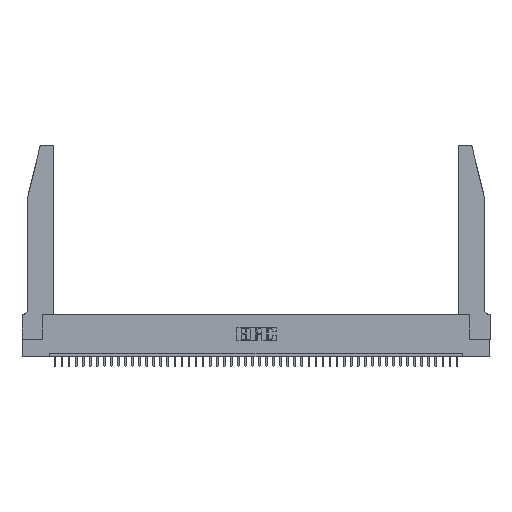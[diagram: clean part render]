
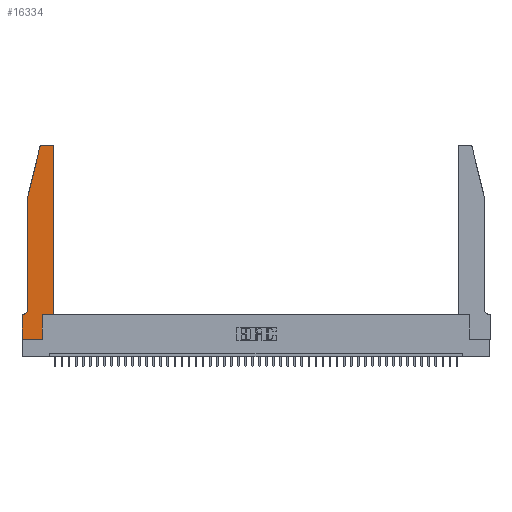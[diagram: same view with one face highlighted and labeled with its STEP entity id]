
A CAD part, top view. The second image highlights one B-rep face of the part: STEP entity #16334.
In plain terms, the highlighted planar face has unit normal (0, 0, 1).
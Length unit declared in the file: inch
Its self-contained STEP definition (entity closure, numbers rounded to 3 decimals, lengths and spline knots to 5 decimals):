
#202 = DIRECTION ( 'NONE',  ( 0., 0., 1. ) ) ;
#338 = CIRCLE ( 'NONE', #2406, 0.03 ) ;
#972 = VECTOR ( 'NONE', #3423, 39.37008 ) ;
#1377 = CARTESIAN_POINT ( 'NONE',  ( 0.2865, 0.35, 0.37 ) ) ;
#1433 = ORIENTED_EDGE ( 'NONE', *, *, #44359, .T. ) ;
#1710 = DIRECTION ( 'NONE',  ( -1., 0., 0. ) ) ;
#1932 = CARTESIAN_POINT ( 'NONE',  ( 0., 0.35, 0.37 ) ) ;
#2041 = CARTESIAN_POINT ( 'NONE',  ( 0.4505, 0.35, 0.37 ) ) ;
#2165 = VECTOR ( 'NONE', #20961, 39.37008 ) ;
#2406 = AXIS2_PLACEMENT_3D ( 'NONE', #21617, #202, #3395 ) ;
#2463 = VERTEX_POINT ( 'NONE', #12196 ) ;
#2534 = CARTESIAN_POINT ( 'NONE',  ( 0., 0., 0.37 ) ) ;
#3395 = DIRECTION ( 'NONE',  ( 1., 0., 0. ) ) ;
#3423 = DIRECTION ( 'NONE',  ( 0., -1., 0. ) ) ;
#3907 = DIRECTION ( 'NONE',  ( -1., 0., 0. ) ) ;
#4202 = DIRECTION ( 'NONE',  ( 1., 0., 0. ) ) ;
#5091 = LINE ( 'NONE', #2041, #32453 ) ;
#5204 = CARTESIAN_POINT ( 'NONE',  ( 0.0755, 2., 0.37 ) ) ;
#5211 = ORIENTED_EDGE ( 'NONE', *, *, #23119, .T. ) ;
#6109 = VERTEX_POINT ( 'NONE', #40522 ) ;
#7480 = LINE ( 'NONE', #2534, #35958 ) ;
#7808 = DIRECTION ( 'NONE',  ( 1., 0., 0. ) ) ;
#8692 = DIRECTION ( 'NONE',  ( 0., 0., 1. ) ) ;
#9276 = DIRECTION ( 'NONE',  ( 0., 1., 0. ) ) ;
#9297 = CARTESIAN_POINT ( 'NONE',  ( 0., 0.35, 0.37 ) ) ;
#9878 = LINE ( 'NONE', #5204, #30496 ) ;
#11547 = EDGE_CURVE ( 'NONE', #17752, #16290, #7480, .T. ) ;
#11912 = DIRECTION ( 'NONE',  ( 0., -1., 0. ) ) ;
#12196 = CARTESIAN_POINT ( 'NONE',  ( 0.4505, 2.72, 0.37 ) ) ;
#12295 = ORIENTED_EDGE ( 'NONE', *, *, #21421, .T. ) ;
#12437 = VERTEX_POINT ( 'NONE', #1377 ) ;
#12793 = CARTESIAN_POINT ( 'NONE',  ( 0.284, 2.72, 0.37 ) ) ;
#13171 = CIRCLE ( 'NONE', #36672, 0.03 ) ;
#13835 = EDGE_CURVE ( 'NONE', #16376, #28984, #25626, .T. ) ;
#14443 = ORIENTED_EDGE ( 'NONE', *, *, #32983, .T. ) ;
#15284 = VERTEX_POINT ( 'NONE', #29966 ) ;
#16290 = VERTEX_POINT ( 'NONE', #25837 ) ;
#16334 = ADVANCED_FACE ( 'NONE', ( #22811 ), #37228, .T. ) ;
#16376 = VERTEX_POINT ( 'NONE', #43990 ) ;
#17752 = VERTEX_POINT ( 'NONE', #31110 ) ;
#18960 = VECTOR ( 'NONE', #21909, 39.37008 ) ;
#19175 = ORIENTED_EDGE ( 'NONE', *, *, #13835, .T. ) ;
#19849 = DIRECTION ( 'NONE',  ( -0.239, -0.971, 0. ) ) ;
#20037 = LINE ( 'NONE', #24501, #972 ) ;
#20463 = CARTESIAN_POINT ( 'NONE',  ( 0.4505, 0.35, 0.37 ) ) ;
#20860 = ORIENTED_EDGE ( 'NONE', *, *, #30473, .T. ) ;
#20961 = DIRECTION ( 'NONE',  ( -1., 0., 0. ) ) ;
#21421 = EDGE_CURVE ( 'NONE', #28984, #17752, #31409, .T. ) ;
#21617 = CARTESIAN_POINT ( 'NONE',  ( 0.4205, 2.72, 0.37 ) ) ;
#21909 = DIRECTION ( 'NONE',  ( 0., 1., 0. ) ) ;
#22383 = EDGE_CURVE ( 'NONE', #44766, #2463, #45265, .T. ) ;
#22584 = EDGE_LOOP ( 'NONE', ( #20860, #5211, #32523, #14443, #23298, #19175, #12295, #41637, #33372, #25308, #46089, #1433 ) ) ;
#22811 = FACE_OUTER_BOUND ( 'NONE', #22584, .T. ) ;
#23119 = EDGE_CURVE ( 'NONE', #30711, #6109, #13171, .T. ) ;
#23289 = DIRECTION ( 'NONE',  ( 1., 0., 0. ) ) ;
#23298 = ORIENTED_EDGE ( 'NONE', *, *, #37552, .T. ) ;
#24154 = VECTOR ( 'NONE', #11912, 39.37008 ) ;
#24501 = CARTESIAN_POINT ( 'NONE',  ( 0.0755, 2., 0.37 ) ) ;
#24625 = LINE ( 'NONE', #43150, #18960 ) ;
#25156 = VECTOR ( 'NONE', #9276, 39.37008 ) ;
#25308 = ORIENTED_EDGE ( 'NONE', *, *, #42397, .T. ) ;
#25626 = LINE ( 'NONE', #35508, #2165 ) ;
#25776 = CARTESIAN_POINT ( 'NONE',  ( 0., 0., 0.37 ) ) ;
#25837 = CARTESIAN_POINT ( 'NONE',  ( 0.2865, 0., 0.37 ) ) ;
#26424 = VERTEX_POINT ( 'NONE', #38576 ) ;
#26479 = EDGE_CURVE ( 'NONE', #16290, #12437, #24625, .T. ) ;
#28166 = LINE ( 'NONE', #28340, #31508 ) ;
#28340 = CARTESIAN_POINT ( 'NONE',  ( 0.2605, 2.75, 0.37 ) ) ;
#28984 = VERTEX_POINT ( 'NONE', #9297 ) ;
#29966 = CARTESIAN_POINT ( 'NONE',  ( 0.4205, 2.75, 0.37 ) ) ;
#30473 = EDGE_CURVE ( 'NONE', #15284, #30711, #28166, .T. ) ;
#30496 = VECTOR ( 'NONE', #19849, 39.37008 ) ;
#30711 = VERTEX_POINT ( 'NONE', #43423 ) ;
#31110 = CARTESIAN_POINT ( 'NONE',  ( 0., 0., 0.37 ) ) ;
#31409 = LINE ( 'NONE', #25776, #24154 ) ;
#31508 = VECTOR ( 'NONE', #1710, 39.37008 ) ;
#31632 = DIRECTION ( 'NONE',  ( 0., 0., 1. ) ) ;
#32453 = VECTOR ( 'NONE', #23289, 39.37008 ) ;
#32523 = ORIENTED_EDGE ( 'NONE', *, *, #45430, .T. ) ;
#32555 = CIRCLE ( 'NONE', #40181, 0.07 ) ;
#32983 = EDGE_CURVE ( 'NONE', #42905, #26424, #20037, .T. ) ;
#33372 = ORIENTED_EDGE ( 'NONE', *, *, #26479, .T. ) ;
#35508 = CARTESIAN_POINT ( 'NONE',  ( 0.0755, 0.35, 0.37 ) ) ;
#35822 = DIRECTION ( 'NONE',  ( 1., 0., 0. ) ) ;
#35958 = VECTOR ( 'NONE', #7808, 39.37008 ) ;
#36061 = CARTESIAN_POINT ( 'NONE',  ( 0.0055, 0.42, 0.37 ) ) ;
#36088 = CARTESIAN_POINT ( 'NONE',  ( 0.4505, 0.35, 0.37 ) ) ;
#36672 = AXIS2_PLACEMENT_3D ( 'NONE', #12793, #8692, #4202 ) ;
#37228 = PLANE ( 'NONE',  #40705 ) ;
#37552 = EDGE_CURVE ( 'NONE', #26424, #16376, #32555, .T. ) ;
#38476 = CARTESIAN_POINT ( 'NONE',  ( 0.0755, 2., 0.37 ) ) ;
#38576 = CARTESIAN_POINT ( 'NONE',  ( 0.0755, 0.42, 0.37 ) ) ;
#40181 = AXIS2_PLACEMENT_3D ( 'NONE', #36061, #43073, #3907 ) ;
#40522 = CARTESIAN_POINT ( 'NONE',  ( 0.25487, 2.72718, 0.37 ) ) ;
#40705 = AXIS2_PLACEMENT_3D ( 'NONE', #1932, #31632, #35822 ) ;
#41637 = ORIENTED_EDGE ( 'NONE', *, *, #11547, .T. ) ;
#42397 = EDGE_CURVE ( 'NONE', #12437, #44766, #5091, .T. ) ;
#42905 = VERTEX_POINT ( 'NONE', #38476 ) ;
#43073 = DIRECTION ( 'NONE',  ( 0., 0., -1. ) ) ;
#43150 = CARTESIAN_POINT ( 'NONE',  ( 0.2865, 0.35, 0.37 ) ) ;
#43423 = CARTESIAN_POINT ( 'NONE',  ( 0.284, 2.75, 0.37 ) ) ;
#43990 = CARTESIAN_POINT ( 'NONE',  ( 0.0055, 0.35, 0.37 ) ) ;
#44359 = EDGE_CURVE ( 'NONE', #2463, #15284, #338, .T. ) ;
#44766 = VERTEX_POINT ( 'NONE', #36088 ) ;
#45265 = LINE ( 'NONE', #20463, #25156 ) ;
#45430 = EDGE_CURVE ( 'NONE', #6109, #42905, #9878, .T. ) ;
#46089 = ORIENTED_EDGE ( 'NONE', *, *, #22383, .T. ) ;
